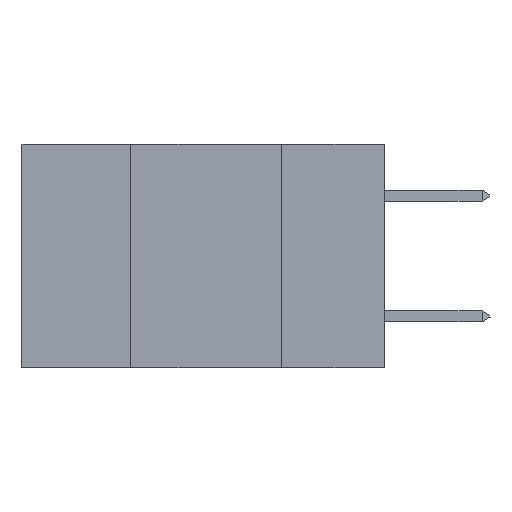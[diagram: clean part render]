
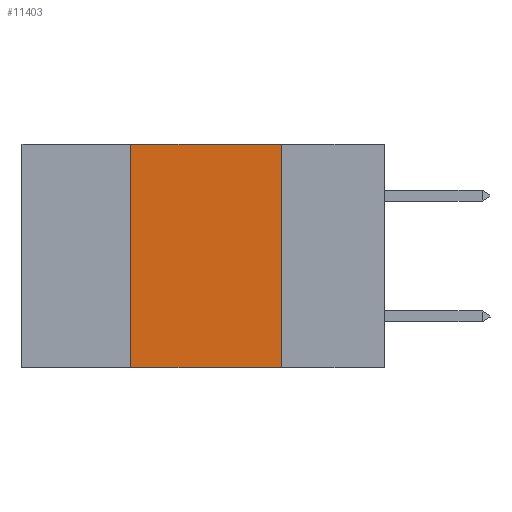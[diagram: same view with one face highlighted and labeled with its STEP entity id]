
A CAD part, left-side view. The second image highlights one B-rep face of the part: STEP entity #11403.
In plain terms, the highlighted planar face has unit normal (-1, 0, 0).
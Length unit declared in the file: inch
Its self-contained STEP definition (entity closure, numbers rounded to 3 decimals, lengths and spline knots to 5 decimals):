
#453 = EDGE_CURVE ( 'NONE', #21870, #20572, #1529, .T. ) ;
#1184 = AXIS2_PLACEMENT_3D ( 'NONE', #14413, #14295, #20078 ) ;
#1529 = LINE ( 'NONE', #3191, #22157 ) ;
#2495 = VECTOR ( 'NONE', #33181, 39.37008 ) ;
#3191 = CARTESIAN_POINT ( 'NONE',  ( 0., 0.17, 0. ) ) ;
#4937 = CARTESIAN_POINT ( 'NONE',  ( 0., 0.42, -0.37 ) ) ;
#5480 = ORIENTED_EDGE ( 'NONE', *, *, #453, .F. ) ;
#5857 = ORIENTED_EDGE ( 'NONE', *, *, #18297, .T. ) ;
#8525 = VECTOR ( 'NONE', #21027, 39.37008 ) ;
#8674 = CARTESIAN_POINT ( 'NONE',  ( 0., 0.6, -0.37 ) ) ;
#9343 = VERTEX_POINT ( 'NONE', #4937 ) ;
#11403 = ADVANCED_FACE ( 'NONE', ( #12288 ), #31435, .F. ) ;
#11965 = LINE ( 'NONE', #8674, #25450 ) ;
#12288 = FACE_OUTER_BOUND ( 'NONE', #29928, .T. ) ;
#14295 = DIRECTION ( 'NONE',  ( 1., 0., 0. ) ) ;
#14413 = CARTESIAN_POINT ( 'NONE',  ( 0., 0.6, 0. ) ) ;
#14690 = DIRECTION ( 'NONE',  ( 0., -1., 0. ) ) ;
#15045 = CARTESIAN_POINT ( 'NONE',  ( 0., 0.17, 0. ) ) ;
#15537 = CARTESIAN_POINT ( 'NONE',  ( 0., 0.17, -0.37 ) ) ;
#15900 = CARTESIAN_POINT ( 'NONE',  ( 0., 0.6, 0. ) ) ;
#17661 = DIRECTION ( 'NONE',  ( 0., 0., -1. ) ) ;
#17771 = LINE ( 'NONE', #15900, #2495 ) ;
#18297 = EDGE_CURVE ( 'NONE', #9343, #20572, #11965, .T. ) ;
#19626 = VERTEX_POINT ( 'NONE', #35148 ) ;
#20078 = DIRECTION ( 'NONE',  ( 0., 0., -1. ) ) ;
#20572 = VERTEX_POINT ( 'NONE', #15537 ) ;
#21027 = DIRECTION ( 'NONE',  ( 0., 0., 1. ) ) ;
#21870 = VERTEX_POINT ( 'NONE', #15045 ) ;
#22157 = VECTOR ( 'NONE', #17661, 39.37008 ) ;
#23943 = ORIENTED_EDGE ( 'NONE', *, *, #26727, .F. ) ;
#25450 = VECTOR ( 'NONE', #14690, 39.37008 ) ;
#26727 = EDGE_CURVE ( 'NONE', #9343, #19626, #33627, .T. ) ;
#29928 = EDGE_LOOP ( 'NONE', ( #5480, #36334, #23943, #5857 ) ) ;
#31435 = PLANE ( 'NONE',  #1184 ) ;
#33181 = DIRECTION ( 'NONE',  ( 0., -1., 0. ) ) ;
#33627 = LINE ( 'NONE', #35327, #8525 ) ;
#35148 = CARTESIAN_POINT ( 'NONE',  ( 0., 0.42, 0. ) ) ;
#35327 = CARTESIAN_POINT ( 'NONE',  ( 0., 0.42, 0. ) ) ;
#35686 = EDGE_CURVE ( 'NONE', #19626, #21870, #17771, .T. ) ;
#36334 = ORIENTED_EDGE ( 'NONE', *, *, #35686, .F. ) ;
